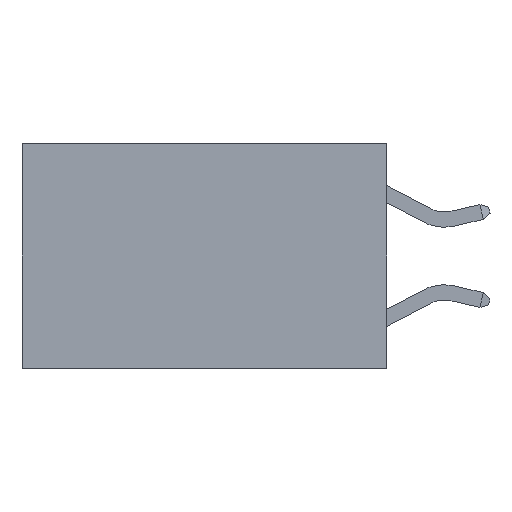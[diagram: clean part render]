
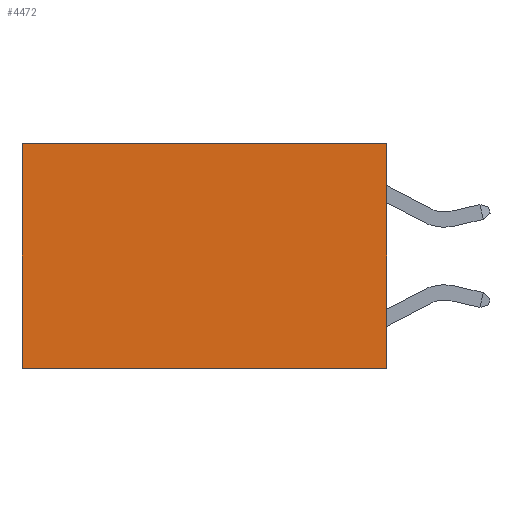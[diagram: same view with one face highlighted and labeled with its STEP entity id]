
A CAD part, left-side view. The second image highlights one B-rep face of the part: STEP entity #4472.
In plain terms, the highlighted planar face has unit normal (-1, 0, 0).
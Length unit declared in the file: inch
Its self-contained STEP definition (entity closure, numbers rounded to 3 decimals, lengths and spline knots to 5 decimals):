
#174 = ORIENTED_EDGE ( 'NONE', *, *, #22989, .F. ) ;
#1450 = VERTEX_POINT ( 'NONE', #18002 ) ;
#2985 = VECTOR ( 'NONE', #21034, 39.37008 ) ;
#3144 = ORIENTED_EDGE ( 'NONE', *, *, #18094, .T. ) ;
#3843 = EDGE_CURVE ( 'NONE', #1450, #11792, #4741, .T. ) ;
#4125 = CARTESIAN_POINT ( 'NONE',  ( 0.2625, 0., 0. ) ) ;
#4239 = ORIENTED_EDGE ( 'NONE', *, *, #3843, .T. ) ;
#4472 = ADVANCED_FACE ( 'NONE', ( #20645 ), #14909, .F. ) ;
#4741 = LINE ( 'NONE', #22092, #26796 ) ;
#5105 = ORIENTED_EDGE ( 'NONE', *, *, #18841, .F. ) ;
#6353 = DIRECTION ( 'NONE',  ( 0., 0., -1. ) ) ;
#10444 = LINE ( 'NONE', #17763, #21288 ) ;
#10445 = VERTEX_POINT ( 'NONE', #13429 ) ;
#11792 = VERTEX_POINT ( 'NONE', #20279 ) ;
#13429 = CARTESIAN_POINT ( 'NONE',  ( 0.2625, 0., 0. ) ) ;
#14204 = LINE ( 'NONE', #14458, #26449 ) ;
#14458 = CARTESIAN_POINT ( 'NONE',  ( 0.2625, 0., 0. ) ) ;
#14909 = PLANE ( 'NONE',  #23276 ) ;
#16547 = EDGE_LOOP ( 'NONE', ( #4239, #174, #5105, #3144 ) ) ;
#16590 = CARTESIAN_POINT ( 'NONE',  ( 0.2625, 0., -0.37 ) ) ;
#16989 = VERTEX_POINT ( 'NONE', #16590 ) ;
#17763 = CARTESIAN_POINT ( 'NONE',  ( 0.2625, 0., -0.37 ) ) ;
#18002 = CARTESIAN_POINT ( 'NONE',  ( 0.2625, 0.6, 0. ) ) ;
#18094 = EDGE_CURVE ( 'NONE', #10445, #1450, #23262, .T. ) ;
#18841 = EDGE_CURVE ( 'NONE', #10445, #16989, #14204, .T. ) ;
#19118 = DIRECTION ( 'NONE',  ( 0., 0., -1. ) ) ;
#20090 = DIRECTION ( 'NONE',  ( 0., 1., 0. ) ) ;
#20279 = CARTESIAN_POINT ( 'NONE',  ( 0.2625, 0.6, -0.37 ) ) ;
#20645 = FACE_OUTER_BOUND ( 'NONE', #16547, .T. ) ;
#21034 = DIRECTION ( 'NONE',  ( 0., 1., 0. ) ) ;
#21288 = VECTOR ( 'NONE', #20090, 39.37008 ) ;
#22092 = CARTESIAN_POINT ( 'NONE',  ( 0.2625, 0.6, 0. ) ) ;
#22989 = EDGE_CURVE ( 'NONE', #16989, #11792, #10444, .T. ) ;
#23262 = LINE ( 'NONE', #23467, #2985 ) ;
#23276 = AXIS2_PLACEMENT_3D ( 'NONE', #4125, #24854, #6353 ) ;
#23467 = CARTESIAN_POINT ( 'NONE',  ( 0.2625, 0., 0. ) ) ;
#24854 = DIRECTION ( 'NONE',  ( 1., 0., 0. ) ) ;
#26449 = VECTOR ( 'NONE', #19118, 39.37008 ) ;
#26796 = VECTOR ( 'NONE', #27887, 39.37008 ) ;
#27887 = DIRECTION ( 'NONE',  ( 0., 0., -1. ) ) ;
